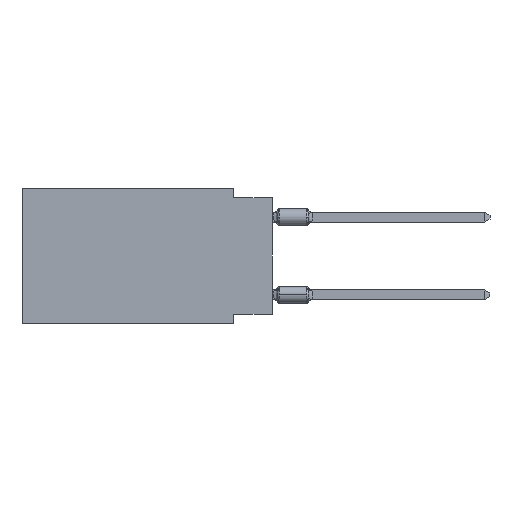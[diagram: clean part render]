
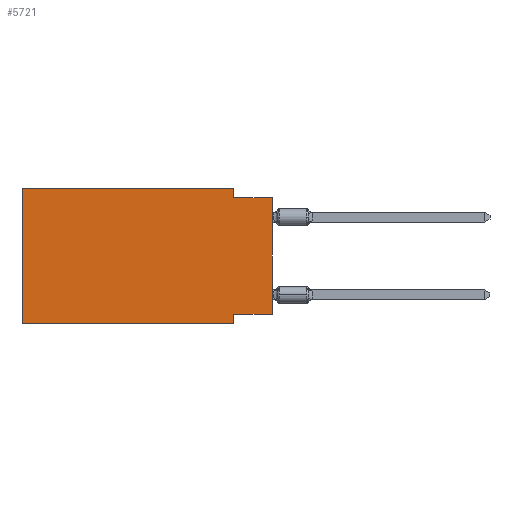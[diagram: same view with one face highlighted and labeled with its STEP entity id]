
A CAD part, left-side view. The second image highlights one B-rep face of the part: STEP entity #5721.
In plain terms, the highlighted planar face has unit normal (-1, 0, 0).
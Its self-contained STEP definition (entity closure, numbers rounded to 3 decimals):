
#255 = ORIENTED_EDGE ( 'NONE', *, *, #10567, .T. ) ;
#267 = CARTESIAN_POINT ( 'NONE',  ( 0., 0., -0.635 ) ) ;
#282 = VECTOR ( 'NONE', #19213, 1000. ) ;
#573 = LINE ( 'NONE', #2218, #17723 ) ;
#804 = CARTESIAN_POINT ( 'NONE',  ( 0., 16.383, -8.89 ) ) ;
#955 = DIRECTION ( 'NONE',  ( 0., 0., -1. ) ) ;
#1016 = LINE ( 'NONE', #804, #1508 ) ;
#1331 = ORIENTED_EDGE ( 'NONE', *, *, #3764, .F. ) ;
#1508 = VECTOR ( 'NONE', #10603, 1000. ) ;
#1762 = CARTESIAN_POINT ( 'NONE',  ( 0., 2.54, -8.89 ) ) ;
#2218 = CARTESIAN_POINT ( 'NONE',  ( 0., 16.383, 0. ) ) ;
#2264 = DIRECTION ( 'NONE',  ( 0., 0., -1. ) ) ;
#2557 = CARTESIAN_POINT ( 'NONE',  ( 0., 0., -8.255 ) ) ;
#2593 = DIRECTION ( 'NONE',  ( 1., 0., 0. ) ) ;
#2638 = ORIENTED_EDGE ( 'NONE', *, *, #12588, .F. ) ;
#3764 = EDGE_CURVE ( 'NONE', #18340, #10272, #573, .T. ) ;
#4094 = VECTOR ( 'NONE', #2264, 1000. ) ;
#4123 = FACE_OUTER_BOUND ( 'NONE', #19966, .T. ) ;
#4354 = CARTESIAN_POINT ( 'NONE',  ( 0., 2.54, -0.635 ) ) ;
#4629 = CARTESIAN_POINT ( 'NONE',  ( 0., 16.383, 0. ) ) ;
#4691 = EDGE_CURVE ( 'NONE', #6312, #10243, #13880, .T. ) ;
#5721 = ADVANCED_FACE ( 'NONE', ( #4123 ), #6073, .F. ) ;
#6006 = ORIENTED_EDGE ( 'NONE', *, *, #20310, .T. ) ;
#6073 = PLANE ( 'NONE',  #11426 ) ;
#6312 = VERTEX_POINT ( 'NONE', #13647 ) ;
#6400 = ORIENTED_EDGE ( 'NONE', *, *, #9130, .F. ) ;
#6617 = DIRECTION ( 'NONE',  ( 0., -1., 0. ) ) ;
#6756 = CARTESIAN_POINT ( 'NONE',  ( 0., 2.54, 0. ) ) ;
#6862 = DIRECTION ( 'NONE',  ( 0., 0., -1. ) ) ;
#6952 = VECTOR ( 'NONE', #6862, 1000. ) ;
#7418 = CARTESIAN_POINT ( 'NONE',  ( 0., 0., -0.635 ) ) ;
#8243 = EDGE_CURVE ( 'NONE', #10243, #16552, #17293, .T. ) ;
#8244 = VECTOR ( 'NONE', #15503, 1000. ) ;
#8593 = CARTESIAN_POINT ( 'NONE',  ( 0., 16.383, -8.89 ) ) ;
#8654 = DIRECTION ( 'NONE',  ( 0., -1., 0. ) ) ;
#9130 = EDGE_CURVE ( 'NONE', #21180, #12201, #20403, .T. ) ;
#9920 = CARTESIAN_POINT ( 'NONE',  ( 0., 2.54, 0. ) ) ;
#10141 = LINE ( 'NONE', #6756, #6952 ) ;
#10167 = VECTOR ( 'NONE', #6617, 1000. ) ;
#10243 = VERTEX_POINT ( 'NONE', #16396 ) ;
#10272 = VERTEX_POINT ( 'NONE', #4629 ) ;
#10567 = EDGE_CURVE ( 'NONE', #18340, #16552, #1016, .T. ) ;
#10603 = DIRECTION ( 'NONE',  ( 0., -1., 0. ) ) ;
#10819 = CARTESIAN_POINT ( 'NONE',  ( 0., 2.54, -8.89 ) ) ;
#11426 = AXIS2_PLACEMENT_3D ( 'NONE', #17518, #2593, #955 ) ;
#12201 = VERTEX_POINT ( 'NONE', #7418 ) ;
#12588 = EDGE_CURVE ( 'NONE', #10272, #16055, #14888, .T. ) ;
#13647 = CARTESIAN_POINT ( 'NONE',  ( 0., 0., -8.255 ) ) ;
#13880 = LINE ( 'NONE', #2557, #282 ) ;
#14166 = DIRECTION ( 'NONE',  ( 0., 0., 1. ) ) ;
#14888 = LINE ( 'NONE', #21529, #10167 ) ;
#15503 = DIRECTION ( 'NONE',  ( 0., 0., 1. ) ) ;
#16055 = VERTEX_POINT ( 'NONE', #9920 ) ;
#16088 = EDGE_CURVE ( 'NONE', #16055, #21180, #10141, .T. ) ;
#16396 = CARTESIAN_POINT ( 'NONE',  ( 0., 2.54, -8.255 ) ) ;
#16552 = VERTEX_POINT ( 'NONE', #10819 ) ;
#16816 = LINE ( 'NONE', #16925, #8244 ) ;
#16925 = CARTESIAN_POINT ( 'NONE',  ( 0., 0., 0. ) ) ;
#17094 = ORIENTED_EDGE ( 'NONE', *, *, #8243, .F. ) ;
#17293 = LINE ( 'NONE', #1762, #4094 ) ;
#17518 = CARTESIAN_POINT ( 'NONE',  ( 0., 16.383, 0. ) ) ;
#17723 = VECTOR ( 'NONE', #14166, 1000. ) ;
#17951 = ORIENTED_EDGE ( 'NONE', *, *, #16088, .F. ) ;
#18340 = VERTEX_POINT ( 'NONE', #8593 ) ;
#19213 = DIRECTION ( 'NONE',  ( 0., 1., 0. ) ) ;
#19966 = EDGE_LOOP ( 'NONE', ( #6006, #6400, #17951, #2638, #1331, #255, #17094, #20960 ) ) ;
#20310 = EDGE_CURVE ( 'NONE', #6312, #12201, #16816, .T. ) ;
#20403 = LINE ( 'NONE', #267, #21158 ) ;
#20960 = ORIENTED_EDGE ( 'NONE', *, *, #4691, .F. ) ;
#21158 = VECTOR ( 'NONE', #8654, 1000. ) ;
#21180 = VERTEX_POINT ( 'NONE', #4354 ) ;
#21529 = CARTESIAN_POINT ( 'NONE',  ( 0., 16.383, 0. ) ) ;
